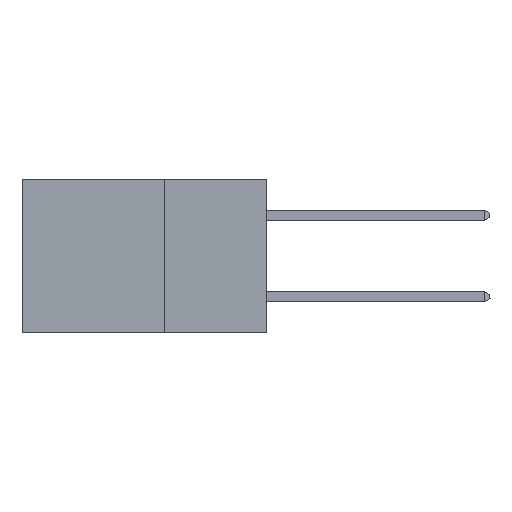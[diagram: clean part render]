
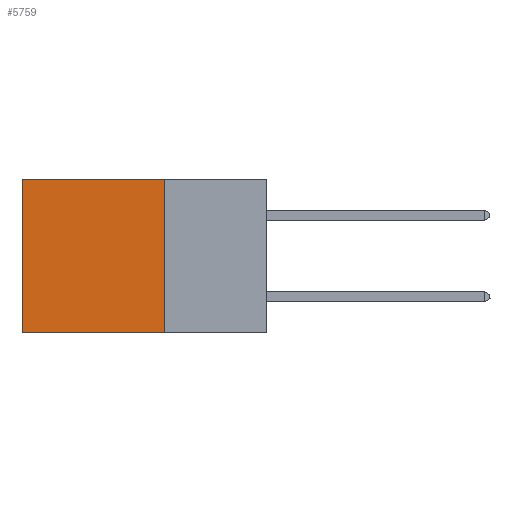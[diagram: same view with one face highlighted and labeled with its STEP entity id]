
A CAD part, left-side view. The second image highlights one B-rep face of the part: STEP entity #5759.
In plain terms, the highlighted planar face has unit normal (-1, 0, 0).
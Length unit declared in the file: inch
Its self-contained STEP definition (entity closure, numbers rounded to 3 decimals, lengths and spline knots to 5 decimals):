
#16 = DIRECTION ( 'NONE',  ( 0., 1., 0. ) ) ;
#219 = EDGE_CURVE ( 'NONE', #2946, #13229, #15478, .T. ) ;
#332 = DIRECTION ( 'NONE',  ( 0., 0., -1. ) ) ;
#490 = EDGE_LOOP ( 'NONE', ( #11137, #13361, #14230, #15509 ) ) ;
#1225 = VECTOR ( 'NONE', #3816, 39.37008 ) ;
#1478 = LINE ( 'NONE', #4838, #7591 ) ;
#2383 = DIRECTION ( 'NONE',  ( 0., 0., -1. ) ) ;
#2529 = CARTESIAN_POINT ( 'NONE',  ( 0.2875, 0.6, -0.375 ) ) ;
#2946 = VERTEX_POINT ( 'NONE', #12547 ) ;
#3816 = DIRECTION ( 'NONE',  ( 0., 1., 0. ) ) ;
#4838 = CARTESIAN_POINT ( 'NONE',  ( 0.2875, 0.25, 0. ) ) ;
#5146 = DIRECTION ( 'NONE',  ( 1., 0., 0. ) ) ;
#5759 = ADVANCED_FACE ( 'NONE', ( #8931 ), #8891, .F. ) ;
#6297 = EDGE_CURVE ( 'NONE', #8243, #2946, #9097, .T. ) ;
#6715 = LINE ( 'NONE', #2529, #12066 ) ;
#7222 = CARTESIAN_POINT ( 'NONE',  ( 0.2875, 0.6, -0.375 ) ) ;
#7382 = CARTESIAN_POINT ( 'NONE',  ( 0.2875, 0.25, -0.375 ) ) ;
#7591 = VECTOR ( 'NONE', #16, 39.37008 ) ;
#8003 = CARTESIAN_POINT ( 'NONE',  ( 0.2875, 0.25, 0. ) ) ;
#8243 = VERTEX_POINT ( 'NONE', #8003 ) ;
#8375 = CARTESIAN_POINT ( 'NONE',  ( 0.2875, 0.6, 0. ) ) ;
#8675 = DIRECTION ( 'NONE',  ( 0., 0., -1. ) ) ;
#8728 = CARTESIAN_POINT ( 'NONE',  ( 0.2875, 0.25, -0.375 ) ) ;
#8891 = PLANE ( 'NONE',  #12626 ) ;
#8931 = FACE_OUTER_BOUND ( 'NONE', #490, .T. ) ;
#9097 = LINE ( 'NONE', #9773, #13851 ) ;
#9773 = CARTESIAN_POINT ( 'NONE',  ( 0.2875, 0.25, -0.375 ) ) ;
#10813 = EDGE_CURVE ( 'NONE', #8243, #11877, #1478, .T. ) ;
#11137 = ORIENTED_EDGE ( 'NONE', *, *, #14035, .T. ) ;
#11877 = VERTEX_POINT ( 'NONE', #8375 ) ;
#12066 = VECTOR ( 'NONE', #332, 39.37008 ) ;
#12547 = CARTESIAN_POINT ( 'NONE',  ( 0.2875, 0.25, -0.375 ) ) ;
#12626 = AXIS2_PLACEMENT_3D ( 'NONE', #8728, #5146, #8675 ) ;
#13229 = VERTEX_POINT ( 'NONE', #7222 ) ;
#13361 = ORIENTED_EDGE ( 'NONE', *, *, #219, .F. ) ;
#13851 = VECTOR ( 'NONE', #2383, 39.37008 ) ;
#14035 = EDGE_CURVE ( 'NONE', #11877, #13229, #6715, .T. ) ;
#14230 = ORIENTED_EDGE ( 'NONE', *, *, #6297, .F. ) ;
#15478 = LINE ( 'NONE', #7382, #1225 ) ;
#15509 = ORIENTED_EDGE ( 'NONE', *, *, #10813, .T. ) ;
